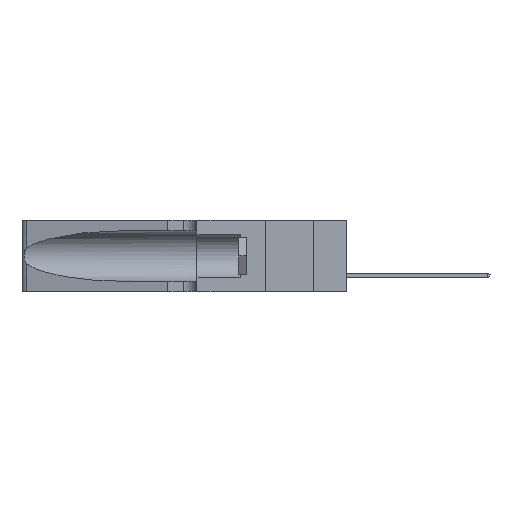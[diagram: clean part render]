
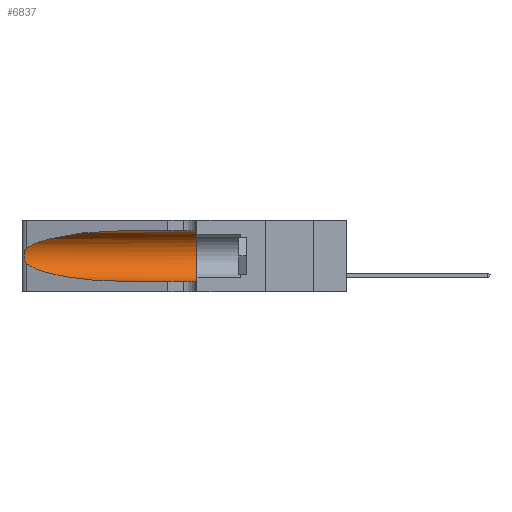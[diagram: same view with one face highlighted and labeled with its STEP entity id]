
A CAD part, left-side view. The second image highlights one B-rep face of the part: STEP entity #6837.
In plain terms, the highlighted cylindrical face has radius 3.308 mm (diameter 6.617 mm), a partial arc.
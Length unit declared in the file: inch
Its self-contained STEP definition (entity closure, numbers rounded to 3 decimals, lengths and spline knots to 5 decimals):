
#82 = EDGE_CURVE ( 'NONE', #45367, #28121, #34847, .T. ) ;
#592 = CARTESIAN_POINT ( 'NONE',  ( 0.25555, 1.22993, 0.14849 ) ) ;
#747 = VERTEX_POINT ( 'NONE', #24775 ) ;
#1072 = CARTESIAN_POINT ( 'NONE',  ( 0.26017, 1.23833, 0.17102 ) ) ;
#1650 = CARTESIAN_POINT ( 'NONE',  ( 0.1305, 0.35, 0.185 ) ) ;
#2252 = CYLINDRICAL_SURFACE ( 'NONE', #31399, 0.13025 ) ;
#3169 = CARTESIAN_POINT ( 'NONE',  ( 0.2373, 1.15595, 0.08982 ) ) ;
#3372 = DIRECTION ( 'NONE',  ( 0., -1., 0. ) ) ;
#3439 = LINE ( 'NONE', #29224, #33021 ) ;
#3790 = CARTESIAN_POINT ( 'NONE',  ( 0.1305, 0.35, 0.31525 ) ) ;
#3842 = CARTESIAN_POINT ( 'NONE',  ( 0.1305, 0.35, 0.05475 ) ) ;
#6032 = DIRECTION ( 'NONE',  ( 0., -1., 0. ) ) ;
#6837 = ADVANCED_FACE ( 'NONE', ( #24440 ), #2252, .F. ) ;
#9170 = CARTESIAN_POINT ( 'NONE',  ( 0.25854, 1.2359, 0.20912 ) ) ;
#9714 =( BOUNDED_CURVE ( )  B_SPLINE_CURVE ( 3, ( #49282, #3169, #19017, #31611 ),
 .UNSPECIFIED., .F., .F. ) 
 B_SPLINE_CURVE_WITH_KNOTS ( ( 4, 4 ),
 ( 3.44316, 4.71239 ),
 .UNSPECIFIED. ) 
 CURVE ( )  GEOMETRIC_REPRESENTATION_ITEM ( )  RATIONAL_B_SPLINE_CURVE ( ( 1., 0.87, 0.87, 1. ) ) 
 REPRESENTATION_ITEM ( '' )  );
#10094 = DIRECTION ( 'NONE',  ( 0., 0., -1. ) ) ;
#10328 = ORIENTED_EDGE ( 'NONE', *, *, #23772, .F. ) ;
#11181 = VERTEX_POINT ( 'NONE', #3790 ) ;
#12437 = CARTESIAN_POINT ( 'NONE',  ( 0.26018, 1.23835, 0.19895 ) ) ;
#12944 = CARTESIAN_POINT ( 'NONE',  ( 0.25555, 1.22994, 0.2215 ) ) ;
#13118 = CARTESIAN_POINT ( 'NONE',  ( 0.25487, 1.22718, 0.22369 ) ) ;
#13777 = CIRCLE ( 'NONE', #21522, 0.13025 ) ;
#15581 = ORIENTED_EDGE ( 'NONE', *, *, #35642, .T. ) ;
#16933 = CARTESIAN_POINT ( 'NONE',  ( 0.25787, 1.23484, 0.2124 ) ) ;
#17044 = CARTESIAN_POINT ( 'NONE',  ( 0.1305, 0.72297, 0.31525 ) ) ;
#18969 = VERTEX_POINT ( 'NONE', #44453 ) ;
#19017 = CARTESIAN_POINT ( 'NONE',  ( 0.18966, 0.96281, 0.05475 ) ) ;
#19233 = B_SPLINE_CURVE_WITH_KNOTS ( 'NONE', 3,
 ( #13118, #12944, #24195, #16933, #9170, #12437, #40724, #32798, #1072, #44480, #20865, #48445, #592, #24857 ),
 .UNSPECIFIED., .F., .F.,
 ( 4, 2, 2, 2, 2, 2, 4 ),
 ( 0., 0.00027, 0.00053, 0.00107, 0.0016, 0.00187, 0.00214 ),
 .UNSPECIFIED. ) ;
#20865 = CARTESIAN_POINT ( 'NONE',  ( 0.25789, 1.23486, 0.15765 ) ) ;
#20982 = CARTESIAN_POINT ( 'NONE',  ( 0.1305, 0.72297, 0.05475 ) ) ;
#21522 = AXIS2_PLACEMENT_3D ( 'NONE', #1650, #24744, #37158 ) ;
#22799 = CARTESIAN_POINT ( 'NONE',  ( 0.25487, 1.22718, 0.22369 ) ) ;
#23772 = EDGE_CURVE ( 'NONE', #40333, #11181, #3439, .T. ) ;
#24195 = CARTESIAN_POINT ( 'NONE',  ( 0.25639, 1.23184, 0.21858 ) ) ;
#24440 = FACE_OUTER_BOUND ( 'NONE', #43138, .T. ) ;
#24744 = DIRECTION ( 'NONE',  ( 0., 1., 0. ) ) ;
#24775 = CARTESIAN_POINT ( 'NONE',  ( 0.25487, 1.22718, 0.22369 ) ) ;
#24857 = CARTESIAN_POINT ( 'NONE',  ( 0.25487, 1.22718, 0.14631 ) ) ;
#28121 = VERTEX_POINT ( 'NONE', #3842 ) ;
#28380 =( BOUNDED_CURVE ( )  B_SPLINE_CURVE ( 3, ( #17044, #34212, #50338, #22799 ),
 .UNSPECIFIED., .F., .F. ) 
 B_SPLINE_CURVE_WITH_KNOTS ( ( 4, 4 ),
 ( 1.5708, 2.84003 ),
 .UNSPECIFIED. ) 
 CURVE ( )  GEOMETRIC_REPRESENTATION_ITEM ( )  RATIONAL_B_SPLINE_CURVE ( ( 1., 0.87, 0.87, 1. ) ) 
 REPRESENTATION_ITEM ( '' )  );
#28866 = ORIENTED_EDGE ( 'NONE', *, *, #82, .T. ) ;
#29224 = CARTESIAN_POINT ( 'NONE',  ( 0.1305, 1.61858, 0.31525 ) ) ;
#29653 = CARTESIAN_POINT ( 'NONE',  ( 0.1305, 1.61858, 0.05475 ) ) ;
#29808 = CARTESIAN_POINT ( 'NONE',  ( 0.1305, 1.61858, 0.185 ) ) ;
#31399 = AXIS2_PLACEMENT_3D ( 'NONE', #29808, #49906, #10094 ) ;
#31611 = CARTESIAN_POINT ( 'NONE',  ( 0.1305, 0.72297, 0.05475 ) ) ;
#32624 = EDGE_CURVE ( 'NONE', #18969, #45367, #9714, .T. ) ;
#32798 = CARTESIAN_POINT ( 'NONE',  ( 0.26075, 1.23896, 0.178 ) ) ;
#33021 = VECTOR ( 'NONE', #3372, 39.37008 ) ;
#34212 = CARTESIAN_POINT ( 'NONE',  ( 0.18966, 0.96281, 0.31525 ) ) ;
#34847 = LINE ( 'NONE', #29653, #49518 ) ;
#35642 = EDGE_CURVE ( 'NONE', #40333, #747, #28380, .T. ) ;
#35701 = EDGE_CURVE ( 'NONE', #11181, #28121, #13777, .T. ) ;
#36366 = ORIENTED_EDGE ( 'NONE', *, *, #39136, .T. ) ;
#36605 = ORIENTED_EDGE ( 'NONE', *, *, #35701, .F. ) ;
#37158 = DIRECTION ( 'NONE',  ( 0., 0., 1. ) ) ;
#39136 = EDGE_CURVE ( 'NONE', #747, #18969, #19233, .T. ) ;
#39609 = CARTESIAN_POINT ( 'NONE',  ( 0.1305, 0.72297, 0.31525 ) ) ;
#40333 = VERTEX_POINT ( 'NONE', #39609 ) ;
#40724 = CARTESIAN_POINT ( 'NONE',  ( 0.26075, 1.23896, 0.19203 ) ) ;
#43138 = EDGE_LOOP ( 'NONE', ( #15581, #36366, #46773, #28866, #36605, #10328 ) ) ;
#44453 = CARTESIAN_POINT ( 'NONE',  ( 0.25487, 1.22718, 0.14631 ) ) ;
#44480 = CARTESIAN_POINT ( 'NONE',  ( 0.25856, 1.23593, 0.16098 ) ) ;
#45367 = VERTEX_POINT ( 'NONE', #20982 ) ;
#46773 = ORIENTED_EDGE ( 'NONE', *, *, #32624, .T. ) ;
#48445 = CARTESIAN_POINT ( 'NONE',  ( 0.25639, 1.23186, 0.15144 ) ) ;
#49282 = CARTESIAN_POINT ( 'NONE',  ( 0.25487, 1.22718, 0.14631 ) ) ;
#49518 = VECTOR ( 'NONE', #6032, 39.37008 ) ;
#49906 = DIRECTION ( 'NONE',  ( 0., -1., 0. ) ) ;
#50338 = CARTESIAN_POINT ( 'NONE',  ( 0.2373, 1.15595, 0.28018 ) ) ;
